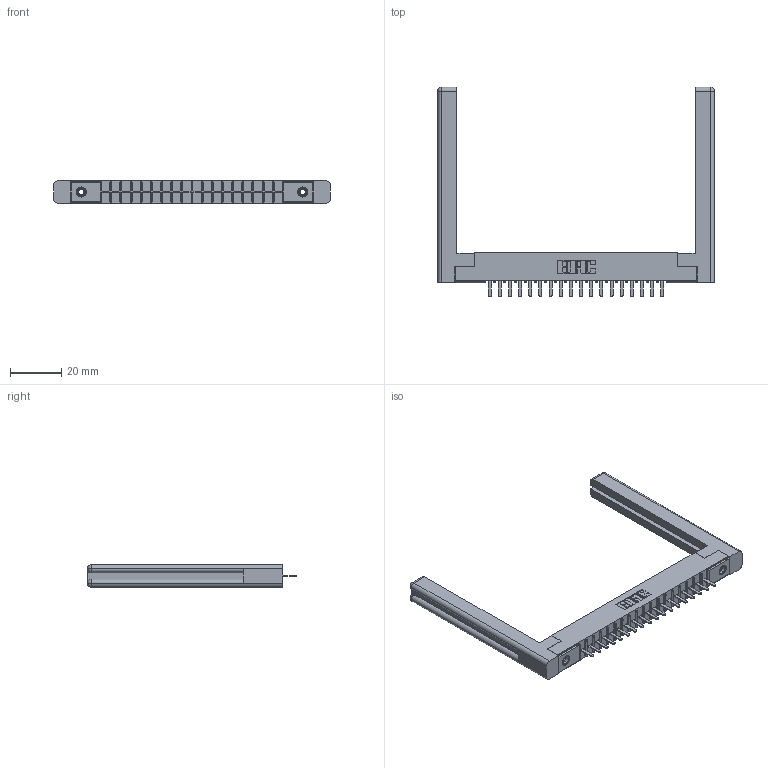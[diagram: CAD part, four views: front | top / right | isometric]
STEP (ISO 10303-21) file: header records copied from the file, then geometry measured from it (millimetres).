
FILE_DESCRIPTION (( 'STEP AP203' ), '1' );
FILE_NAME ('356-018-420-158.STEP', '2020-09-23T13:32:57', ( '' ), ( '' ), 'SwSTEP 2.0', 'SolidWorks 2020', '' );
FILE_SCHEMA (( 'CONFIG_CONTROL_DESIGN' ));
Length unit declared in the file: inch
Products named in the file (5): 306 Part_.156 Dia; 306-290-001_120; 356-018-420-158; 307-220-058; 345-250-001_345-250-001-102
Assembly tree (23 placements, depth 2):
  356-018-420-158
    306 Part_.156 Dia
    306-290-001_120  x18
    345-250-001_345-250-001-102  x2
    307-220-058  x2
Bounding box: 107.95 x 81.76 x 8.71 mm (x, y, z)
Volume: 15009.9 mm3; surface area: 16063.6 mm2
Topology: 23 solids, 23 shells, 1518 faces, 4216 edges, 2700 vertices
Faces by surface type: plane 998, cylinder 424, sphere 72, cone 12, torus 12
Entity records: 22484 total; most frequent: CARTESIAN_POINT 3780, ORIENTED_EDGE 3686, DIRECTION 3685, EDGE_CURVE 1843, LINE 1423, VECTOR 1423, VERTEX_POINT 1172, AXIS2_PLACEMENT_3D 1131
